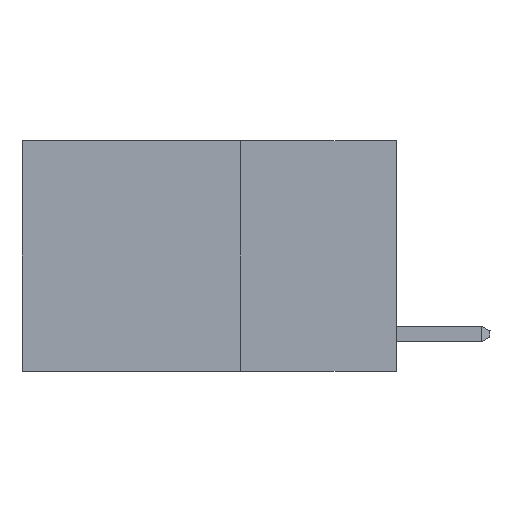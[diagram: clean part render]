
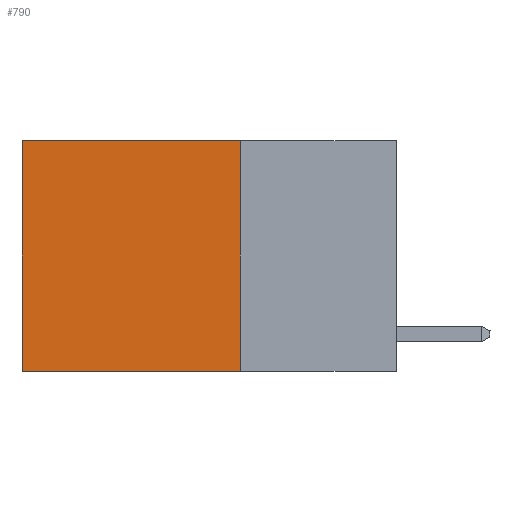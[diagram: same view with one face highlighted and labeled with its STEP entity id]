
A CAD part, left-side view. The second image highlights one B-rep face of the part: STEP entity #790.
In plain terms, the highlighted planar face has unit normal (-1, 0, 0).
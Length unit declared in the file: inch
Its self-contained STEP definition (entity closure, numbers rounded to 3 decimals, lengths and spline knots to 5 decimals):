
#7 = VECTOR ( 'NONE', #12268, 39.37008 ) ;
#348 = CARTESIAN_POINT ( 'NONE',  ( 0.2625, 0.6, 0. ) ) ;
#790 = ADVANCED_FACE ( 'NONE', ( #5689 ), #4975, .F. ) ;
#1405 = EDGE_LOOP ( 'NONE', ( #9714, #9604, #9462, #9317 ) ) ;
#2775 = DIRECTION ( 'NONE',  ( 0., 1., 0. ) ) ;
#3054 = DIRECTION ( 'NONE',  ( 0., 0., -1. ) ) ;
#3370 = CARTESIAN_POINT ( 'NONE',  ( 0.2625, 0.25, -0.37 ) ) ;
#3715 = EDGE_CURVE ( 'NONE', #4710, #8276, #5911, .T. ) ;
#3906 = LINE ( 'NONE', #8062, #9007 ) ;
#3956 = LINE ( 'NONE', #5181, #11515 ) ;
#4311 = CARTESIAN_POINT ( 'NONE',  ( 0.2625, 0.6, -0.37 ) ) ;
#4710 = VERTEX_POINT ( 'NONE', #348 ) ;
#4975 = PLANE ( 'NONE',  #10808 ) ;
#5141 = DIRECTION ( 'NONE',  ( 0., 0., -1. ) ) ;
#5181 = CARTESIAN_POINT ( 'NONE',  ( 0.2625, 0.25, 0. ) ) ;
#5689 = FACE_OUTER_BOUND ( 'NONE', #1405, .T. ) ;
#5911 = LINE ( 'NONE', #9208, #8060 ) ;
#6518 = CARTESIAN_POINT ( 'NONE',  ( 0.2625, 0.25, -0.37 ) ) ;
#6625 = EDGE_CURVE ( 'NONE', #8772, #6750, #3956, .T. ) ;
#6750 = VERTEX_POINT ( 'NONE', #3370 ) ;
#6883 = CARTESIAN_POINT ( 'NONE',  ( 0.2625, 0.25, 0. ) ) ;
#8060 = VECTOR ( 'NONE', #8309, 39.37008 ) ;
#8062 = CARTESIAN_POINT ( 'NONE',  ( 0.2625, 0.25, 0. ) ) ;
#8276 = VERTEX_POINT ( 'NONE', #4311 ) ;
#8309 = DIRECTION ( 'NONE',  ( 0., 0., -1. ) ) ;
#8772 = VERTEX_POINT ( 'NONE', #6883 ) ;
#8836 = EDGE_CURVE ( 'NONE', #8772, #4710, #3906, .T. ) ;
#9007 = VECTOR ( 'NONE', #2775, 39.37008 ) ;
#9208 = CARTESIAN_POINT ( 'NONE',  ( 0.2625, 0.6, 0. ) ) ;
#9311 = DIRECTION ( 'NONE',  ( 1., 0., 0. ) ) ;
#9317 = ORIENTED_EDGE ( 'NONE', *, *, #8836, .T. ) ;
#9462 = ORIENTED_EDGE ( 'NONE', *, *, #6625, .F. ) ;
#9604 = ORIENTED_EDGE ( 'NONE', *, *, #12132, .F. ) ;
#9714 = ORIENTED_EDGE ( 'NONE', *, *, #3715, .T. ) ;
#10749 = CARTESIAN_POINT ( 'NONE',  ( 0.2625, 0.25, 0. ) ) ;
#10808 = AXIS2_PLACEMENT_3D ( 'NONE', #10749, #9311, #3054 ) ;
#10843 = LINE ( 'NONE', #6518, #7 ) ;
#11515 = VECTOR ( 'NONE', #5141, 39.37008 ) ;
#12132 = EDGE_CURVE ( 'NONE', #6750, #8276, #10843, .T. ) ;
#12268 = DIRECTION ( 'NONE',  ( 0., 1., 0. ) ) ;
